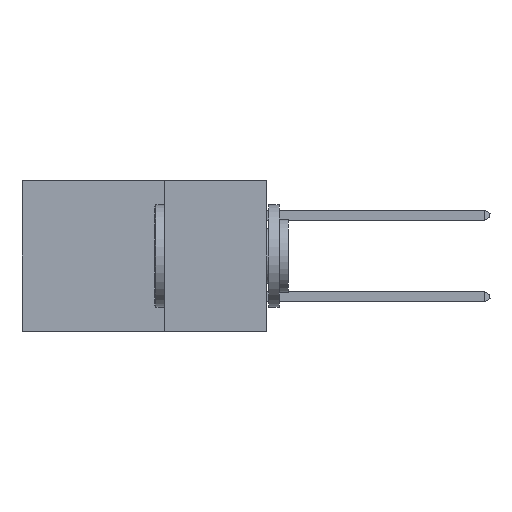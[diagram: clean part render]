
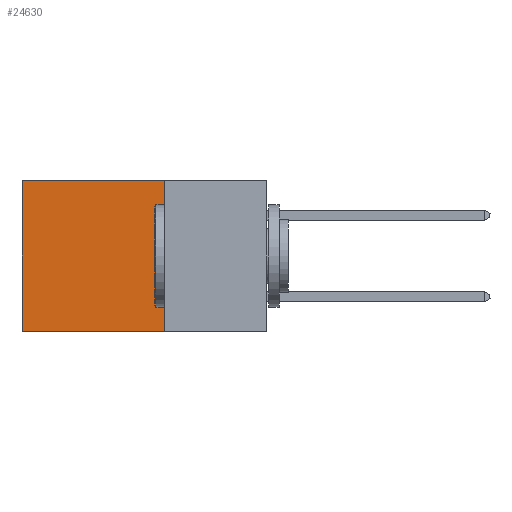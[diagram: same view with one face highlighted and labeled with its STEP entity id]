
A CAD part, left-side view. The second image highlights one B-rep face of the part: STEP entity #24630.
In plain terms, the highlighted planar face has unit normal (-1, 0, 0).
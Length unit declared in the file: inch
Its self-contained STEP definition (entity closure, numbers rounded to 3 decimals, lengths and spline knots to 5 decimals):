
#756 = VECTOR ( 'NONE', #3038, 39.37008 ) ;
#1538 = DIRECTION ( 'NONE',  ( 0., 0., -1. ) ) ;
#3038 = DIRECTION ( 'NONE',  ( 0., 1., 0. ) ) ;
#3988 = CARTESIAN_POINT ( 'NONE',  ( 0.2875, 0.25, -0.37 ) ) ;
#5076 = EDGE_LOOP ( 'NONE', ( #32362, #20515, #10342, #11882 ) ) ;
#5173 = CARTESIAN_POINT ( 'NONE',  ( 0.2875, 0.25, -0.37 ) ) ;
#5841 = CARTESIAN_POINT ( 'NONE',  ( 0.2875, 0.25, 0. ) ) ;
#9781 = CARTESIAN_POINT ( 'NONE',  ( 0.2875, 0.6, 0. ) ) ;
#10321 = VECTOR ( 'NONE', #28000, 39.37008 ) ;
#10342 = ORIENTED_EDGE ( 'NONE', *, *, #36852, .F. ) ;
#10908 = VECTOR ( 'NONE', #25468, 39.37008 ) ;
#11335 = VERTEX_POINT ( 'NONE', #21616 ) ;
#11882 = ORIENTED_EDGE ( 'NONE', *, *, #18095, .T. ) ;
#12750 = PLANE ( 'NONE',  #31107 ) ;
#14554 = EDGE_CURVE ( 'NONE', #26339, #31074, #34533, .T. ) ;
#18095 = EDGE_CURVE ( 'NONE', #11335, #26339, #24425, .T. ) ;
#20515 = ORIENTED_EDGE ( 'NONE', *, *, #35401, .F. ) ;
#21616 = CARTESIAN_POINT ( 'NONE',  ( 0.2875, 0.25, 0. ) ) ;
#21756 = CARTESIAN_POINT ( 'NONE',  ( 0.2875, 0.25, 0. ) ) ;
#22579 = LINE ( 'NONE', #28251, #10321 ) ;
#24425 = LINE ( 'NONE', #5841, #756 ) ;
#24522 = DIRECTION ( 'NONE',  ( 1., 0., 0. ) ) ;
#24630 = ADVANCED_FACE ( 'NONE', ( #31576 ), #12750, .F. ) ;
#25468 = DIRECTION ( 'NONE',  ( 0., 1., 0. ) ) ;
#26339 = VERTEX_POINT ( 'NONE', #28023 ) ;
#28000 = DIRECTION ( 'NONE',  ( 0., 0., -1. ) ) ;
#28023 = CARTESIAN_POINT ( 'NONE',  ( 0.2875, 0.6, 0. ) ) ;
#28251 = CARTESIAN_POINT ( 'NONE',  ( 0.2875, 0.25, 0. ) ) ;
#28600 = LINE ( 'NONE', #5173, #10908 ) ;
#31074 = VERTEX_POINT ( 'NONE', #32553 ) ;
#31107 = AXIS2_PLACEMENT_3D ( 'NONE', #21756, #24522, #1538 ) ;
#31576 = FACE_OUTER_BOUND ( 'NONE', #5076, .T. ) ;
#32362 = ORIENTED_EDGE ( 'NONE', *, *, #14554, .T. ) ;
#32553 = CARTESIAN_POINT ( 'NONE',  ( 0.2875, 0.6, -0.37 ) ) ;
#32955 = DIRECTION ( 'NONE',  ( 0., 0., -1. ) ) ;
#34533 = LINE ( 'NONE', #9781, #36374 ) ;
#35401 = EDGE_CURVE ( 'NONE', #37045, #31074, #28600, .T. ) ;
#36374 = VECTOR ( 'NONE', #32955, 39.37008 ) ;
#36852 = EDGE_CURVE ( 'NONE', #11335, #37045, #22579, .T. ) ;
#37045 = VERTEX_POINT ( 'NONE', #3988 ) ;
